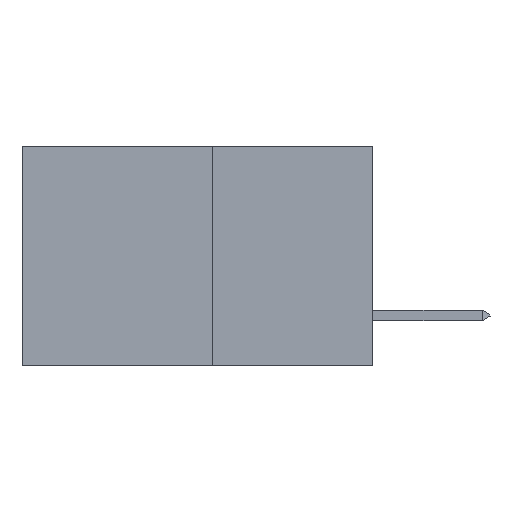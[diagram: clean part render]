
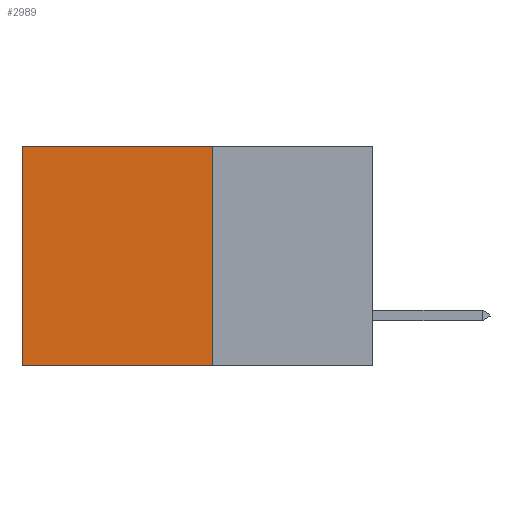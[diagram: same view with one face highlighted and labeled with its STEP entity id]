
A CAD part, left-side view. The second image highlights one B-rep face of the part: STEP entity #2989.
In plain terms, the highlighted planar face has unit normal (-1, 0, 0).
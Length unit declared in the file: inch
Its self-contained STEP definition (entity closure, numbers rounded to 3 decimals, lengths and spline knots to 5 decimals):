
#93 = ORIENTED_EDGE ( 'NONE', *, *, #2015, .T. ) ;
#113 = CARTESIAN_POINT ( 'NONE',  ( 0.277, 0.59, 0. ) ) ;
#320 = DIRECTION ( 'NONE',  ( 0., 1., 0. ) ) ;
#624 = DIRECTION ( 'NONE',  ( 0., 0., -1. ) ) ;
#1104 = ORIENTED_EDGE ( 'NONE', *, *, #2051, .F. ) ;
#1503 = CARTESIAN_POINT ( 'NONE',  ( 0.277, 0.27, 0. ) ) ;
#1717 = DIRECTION ( 'NONE',  ( 0., 0., -1. ) ) ;
#2015 = EDGE_CURVE ( 'NONE', #4399, #10503, #11110, .T. ) ;
#2051 = EDGE_CURVE ( 'NONE', #2206, #10503, #13430, .T. ) ;
#2206 = VERTEX_POINT ( 'NONE', #7963 ) ;
#2359 = CARTESIAN_POINT ( 'NONE',  ( 0.277, 0.59, -0.37 ) ) ;
#2514 = FACE_OUTER_BOUND ( 'NONE', #2578, .T. ) ;
#2578 = EDGE_LOOP ( 'NONE', ( #93, #1104, #7990, #9948 ) ) ;
#2835 = VECTOR ( 'NONE', #1717, 39.37008 ) ;
#2989 = ADVANCED_FACE ( 'NONE', ( #2514 ), #7763, .F. ) ;
#3129 = CARTESIAN_POINT ( 'NONE',  ( 0.277, 0.27, -0.37 ) ) ;
#4072 = VECTOR ( 'NONE', #10855, 39.37008 ) ;
#4331 = EDGE_CURVE ( 'NONE', #10443, #2206, #11360, .T. ) ;
#4399 = VERTEX_POINT ( 'NONE', #113 ) ;
#5203 = EDGE_CURVE ( 'NONE', #10443, #4399, #7704, .T. ) ;
#7704 = LINE ( 'NONE', #1503, #4072 ) ;
#7763 = PLANE ( 'NONE',  #11592 ) ;
#7963 = CARTESIAN_POINT ( 'NONE',  ( 0.277, 0.27, -0.37 ) ) ;
#7990 = ORIENTED_EDGE ( 'NONE', *, *, #4331, .F. ) ;
#8423 = VECTOR ( 'NONE', #624, 39.37008 ) ;
#8613 = CARTESIAN_POINT ( 'NONE',  ( 0.277, 0.27, 0. ) ) ;
#8651 = DIRECTION ( 'NONE',  ( 1., 0., 0. ) ) ;
#8840 = CARTESIAN_POINT ( 'NONE',  ( 0.277, 0.27, -0.37 ) ) ;
#9834 = DIRECTION ( 'NONE',  ( 0., 0., -1. ) ) ;
#9948 = ORIENTED_EDGE ( 'NONE', *, *, #5203, .T. ) ;
#10151 = VECTOR ( 'NONE', #320, 39.37008 ) ;
#10443 = VERTEX_POINT ( 'NONE', #8613 ) ;
#10503 = VERTEX_POINT ( 'NONE', #10724 ) ;
#10724 = CARTESIAN_POINT ( 'NONE',  ( 0.277, 0.59, -0.37 ) ) ;
#10855 = DIRECTION ( 'NONE',  ( 0., 1., 0. ) ) ;
#11110 = LINE ( 'NONE', #2359, #8423 ) ;
#11360 = LINE ( 'NONE', #8840, #2835 ) ;
#11592 = AXIS2_PLACEMENT_3D ( 'NONE', #3129, #8651, #9834 ) ;
#12646 = CARTESIAN_POINT ( 'NONE',  ( 0.277, 0.27, -0.37 ) ) ;
#13430 = LINE ( 'NONE', #12646, #10151 ) ;
